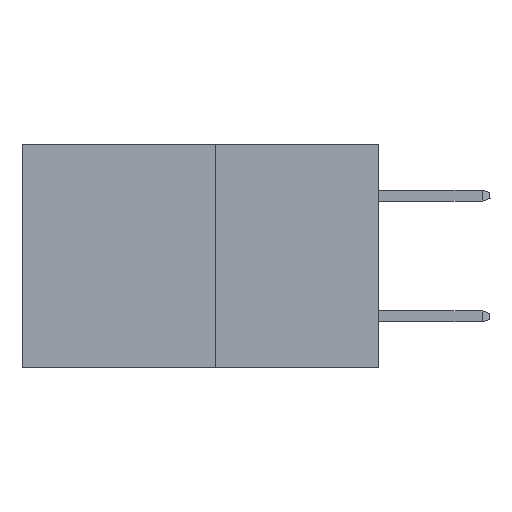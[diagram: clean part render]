
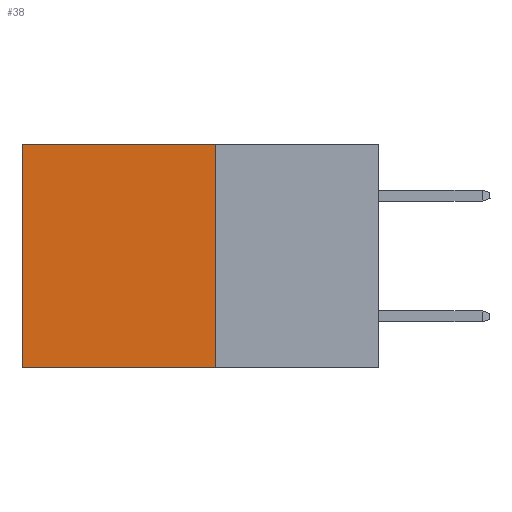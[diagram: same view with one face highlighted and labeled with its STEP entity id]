
A CAD part, left-side view. The second image highlights one B-rep face of the part: STEP entity #38.
In plain terms, the highlighted planar face has unit normal (-1, 0, 0).
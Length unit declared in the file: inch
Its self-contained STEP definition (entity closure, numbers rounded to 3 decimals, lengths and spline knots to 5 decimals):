
#38 = ADVANCED_FACE ( 'NONE', ( #19435 ), #13924, .F. ) ;
#669 = VERTEX_POINT ( 'NONE', #13455 ) ;
#1361 = EDGE_CURVE ( 'NONE', #8851, #669, #17502, .T. ) ;
#1362 = ORIENTED_EDGE ( 'NONE', *, *, #17544, .F. ) ;
#1939 = AXIS2_PLACEMENT_3D ( 'NONE', #7219, #2741, #13057 ) ;
#2741 = DIRECTION ( 'NONE',  ( 1., 0., 0. ) ) ;
#2867 = CARTESIAN_POINT ( 'NONE',  ( 0.277, 0.27, 0. ) ) ;
#2876 = CARTESIAN_POINT ( 'NONE',  ( 0.277, 0.59, -0.37 ) ) ;
#3074 = CARTESIAN_POINT ( 'NONE',  ( 0.277, 0.27, 0. ) ) ;
#3198 = LINE ( 'NONE', #11308, #7290 ) ;
#3691 = DIRECTION ( 'NONE',  ( 0., 0., -1. ) ) ;
#6258 = DIRECTION ( 'NONE',  ( 0., 1., 0. ) ) ;
#6424 = LINE ( 'NONE', #12302, #20152 ) ;
#6901 = VERTEX_POINT ( 'NONE', #2876 ) ;
#7101 = DIRECTION ( 'NONE',  ( 0., 1., 0. ) ) ;
#7219 = CARTESIAN_POINT ( 'NONE',  ( 0.277, 0.27, -0.37 ) ) ;
#7290 = VECTOR ( 'NONE', #13017, 39.37008 ) ;
#7636 = ORIENTED_EDGE ( 'NONE', *, *, #1361, .T. ) ;
#8851 = VERTEX_POINT ( 'NONE', #2867 ) ;
#9499 = EDGE_CURVE ( 'NONE', #8851, #10619, #6424, .T. ) ;
#10619 = VERTEX_POINT ( 'NONE', #21898 ) ;
#11108 = LINE ( 'NONE', #16583, #20212 ) ;
#11308 = CARTESIAN_POINT ( 'NONE',  ( 0.277, 0.59, -0.37 ) ) ;
#12302 = CARTESIAN_POINT ( 'NONE',  ( 0.277, 0.27, -0.37 ) ) ;
#12387 = VECTOR ( 'NONE', #7101, 39.37008 ) ;
#13017 = DIRECTION ( 'NONE',  ( 0., 0., -1. ) ) ;
#13057 = DIRECTION ( 'NONE',  ( 0., 0., -1. ) ) ;
#13455 = CARTESIAN_POINT ( 'NONE',  ( 0.277, 0.59, 0. ) ) ;
#13924 = PLANE ( 'NONE',  #1939 ) ;
#14595 = ORIENTED_EDGE ( 'NONE', *, *, #18198, .T. ) ;
#14912 = EDGE_LOOP ( 'NONE', ( #14595, #1362, #19722, #7636 ) ) ;
#16583 = CARTESIAN_POINT ( 'NONE',  ( 0.277, 0.27, -0.37 ) ) ;
#17502 = LINE ( 'NONE', #3074, #12387 ) ;
#17544 = EDGE_CURVE ( 'NONE', #10619, #6901, #11108, .T. ) ;
#18198 = EDGE_CURVE ( 'NONE', #669, #6901, #3198, .T. ) ;
#19435 = FACE_OUTER_BOUND ( 'NONE', #14912, .T. ) ;
#19722 = ORIENTED_EDGE ( 'NONE', *, *, #9499, .F. ) ;
#20152 = VECTOR ( 'NONE', #3691, 39.37008 ) ;
#20212 = VECTOR ( 'NONE', #6258, 39.37008 ) ;
#21898 = CARTESIAN_POINT ( 'NONE',  ( 0.277, 0.27, -0.37 ) ) ;
